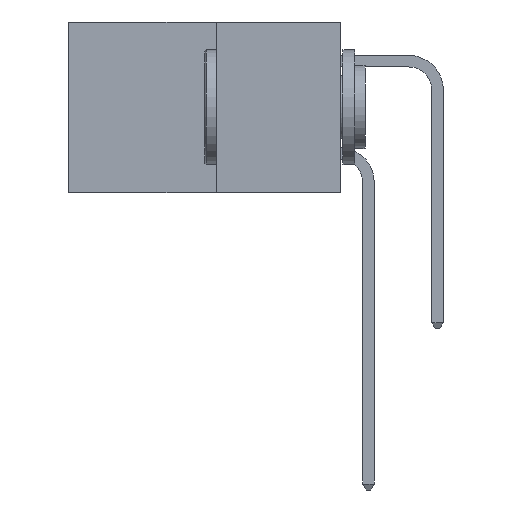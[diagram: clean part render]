
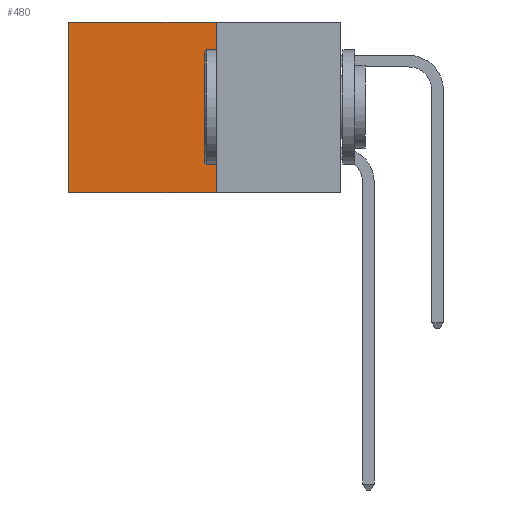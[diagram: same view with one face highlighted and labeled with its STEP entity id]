
A CAD part, left-side view. The second image highlights one B-rep face of the part: STEP entity #480.
In plain terms, the highlighted planar face has unit normal (-1, 0, 0).
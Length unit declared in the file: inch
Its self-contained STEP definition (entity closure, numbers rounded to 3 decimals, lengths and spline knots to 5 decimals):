
#480 = ADVANCED_FACE ( 'NONE', ( #1894 ), #12343, .F. ) ;
#603 = VERTEX_POINT ( 'NONE', #23693 ) ;
#694 = VECTOR ( 'NONE', #10759, 39.37008 ) ;
#871 = CARTESIAN_POINT ( 'NONE',  ( 0.277, 0.59, -0.37 ) ) ;
#1894 = FACE_OUTER_BOUND ( 'NONE', #8917, .T. ) ;
#2888 = DIRECTION ( 'NONE',  ( 0., 0., -1. ) ) ;
#2895 = VECTOR ( 'NONE', #2888, 39.37008 ) ;
#4562 = DIRECTION ( 'NONE',  ( 0., 0., -1. ) ) ;
#4644 = DIRECTION ( 'NONE',  ( 1., 0., 0. ) ) ;
#5341 = EDGE_CURVE ( 'NONE', #12336, #8220, #25295, .T. ) ;
#5883 = CARTESIAN_POINT ( 'NONE',  ( 0.277, 0.27, -0.37 ) ) ;
#6037 = CARTESIAN_POINT ( 'NONE',  ( 0.277, 0.59, 0. ) ) ;
#6375 = CARTESIAN_POINT ( 'NONE',  ( 0.277, 0.27, -0.37 ) ) ;
#7302 = VECTOR ( 'NONE', #23696, 39.37008 ) ;
#8220 = VERTEX_POINT ( 'NONE', #6037 ) ;
#8917 = EDGE_LOOP ( 'NONE', ( #17773, #23644, #13696, #19002 ) ) ;
#9791 = CARTESIAN_POINT ( 'NONE',  ( 0.277, 0.27, -0.37 ) ) ;
#10759 = DIRECTION ( 'NONE',  ( 0., 1., 0. ) ) ;
#10872 = CARTESIAN_POINT ( 'NONE',  ( 0.277, 0.27, 0. ) ) ;
#11914 = EDGE_CURVE ( 'NONE', #8220, #603, #13522, .T. ) ;
#12095 = VECTOR ( 'NONE', #19855, 39.37008 ) ;
#12336 = VERTEX_POINT ( 'NONE', #21867 ) ;
#12343 = PLANE ( 'NONE',  #13382 ) ;
#12606 = LINE ( 'NONE', #9791, #7302 ) ;
#12950 = EDGE_CURVE ( 'NONE', #19722, #603, #21440, .T. ) ;
#13382 = AXIS2_PLACEMENT_3D ( 'NONE', #24638, #4644, #4562 ) ;
#13522 = LINE ( 'NONE', #871, #2895 ) ;
#13696 = ORIENTED_EDGE ( 'NONE', *, *, #15127, .F. ) ;
#15127 = EDGE_CURVE ( 'NONE', #12336, #19722, #12606, .T. ) ;
#17773 = ORIENTED_EDGE ( 'NONE', *, *, #11914, .T. ) ;
#19002 = ORIENTED_EDGE ( 'NONE', *, *, #5341, .T. ) ;
#19722 = VERTEX_POINT ( 'NONE', #6375 ) ;
#19855 = DIRECTION ( 'NONE',  ( 0., 1., 0. ) ) ;
#21440 = LINE ( 'NONE', #5883, #12095 ) ;
#21867 = CARTESIAN_POINT ( 'NONE',  ( 0.277, 0.27, 0. ) ) ;
#23644 = ORIENTED_EDGE ( 'NONE', *, *, #12950, .F. ) ;
#23693 = CARTESIAN_POINT ( 'NONE',  ( 0.277, 0.59, -0.37 ) ) ;
#23696 = DIRECTION ( 'NONE',  ( 0., 0., -1. ) ) ;
#24638 = CARTESIAN_POINT ( 'NONE',  ( 0.277, 0.27, -0.37 ) ) ;
#25295 = LINE ( 'NONE', #10872, #694 ) ;
